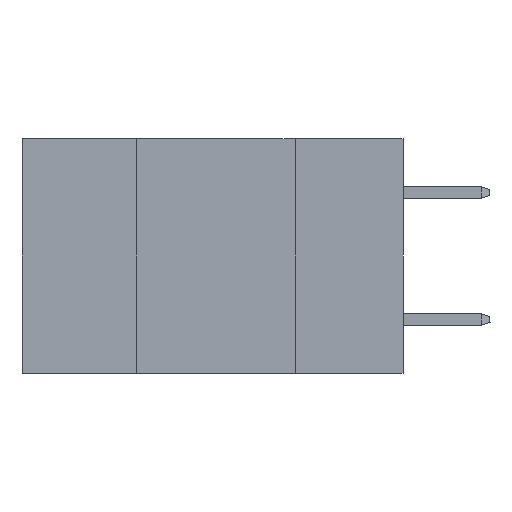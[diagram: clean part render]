
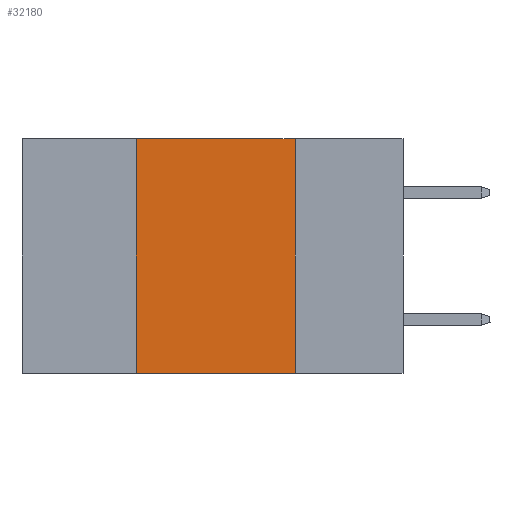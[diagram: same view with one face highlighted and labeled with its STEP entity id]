
A CAD part, left-side view. The second image highlights one B-rep face of the part: STEP entity #32180.
In plain terms, the highlighted planar face has unit normal (-1, 0, 0).
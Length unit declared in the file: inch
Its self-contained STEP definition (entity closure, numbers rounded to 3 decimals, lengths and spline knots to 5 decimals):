
#2008 = VERTEX_POINT ( 'NONE', #32092 ) ;
#3307 = CARTESIAN_POINT ( 'NONE',  ( 0., 0.17, 0. ) ) ;
#3973 = ORIENTED_EDGE ( 'NONE', *, *, #20197, .F. ) ;
#4289 = VERTEX_POINT ( 'NONE', #24339 ) ;
#4741 = LINE ( 'NONE', #33515, #11159 ) ;
#5116 = DIRECTION ( 'NONE',  ( 1., 0., 0. ) ) ;
#5204 = VECTOR ( 'NONE', #11372, 39.37008 ) ;
#5494 = DIRECTION ( 'NONE',  ( 0., -1., 0. ) ) ;
#6930 = CARTESIAN_POINT ( 'NONE',  ( 0., 0.6, -0.37 ) ) ;
#7945 = EDGE_CURVE ( 'NONE', #23927, #22514, #4741, .T. ) ;
#10489 = ORIENTED_EDGE ( 'NONE', *, *, #19503, .F. ) ;
#11159 = VECTOR ( 'NONE', #19785, 39.37008 ) ;
#11293 = VECTOR ( 'NONE', #5494, 39.37008 ) ;
#11372 = DIRECTION ( 'NONE',  ( 0., 0., -1. ) ) ;
#11696 = LINE ( 'NONE', #3307, #5204 ) ;
#14793 = LINE ( 'NONE', #6930, #11293 ) ;
#15014 = ORIENTED_EDGE ( 'NONE', *, *, #7945, .F. ) ;
#15033 = DIRECTION ( 'NONE',  ( 0., 0., -1. ) ) ;
#15169 = DIRECTION ( 'NONE',  ( 0., -1., 0. ) ) ;
#17349 = AXIS2_PLACEMENT_3D ( 'NONE', #28578, #5116, #15033 ) ;
#17660 = ORIENTED_EDGE ( 'NONE', *, *, #23368, .T. ) ;
#18107 = PLANE ( 'NONE',  #17349 ) ;
#19369 = VECTOR ( 'NONE', #15169, 39.37008 ) ;
#19503 = EDGE_CURVE ( 'NONE', #22514, #2008, #22879, .T. ) ;
#19785 = DIRECTION ( 'NONE',  ( 0., 0., 1. ) ) ;
#20197 = EDGE_CURVE ( 'NONE', #2008, #4289, #11696, .T. ) ;
#22514 = VERTEX_POINT ( 'NONE', #22914 ) ;
#22879 = LINE ( 'NONE', #33334, #19369 ) ;
#22914 = CARTESIAN_POINT ( 'NONE',  ( 0., 0.42, 0. ) ) ;
#23368 = EDGE_CURVE ( 'NONE', #23927, #4289, #14793, .T. ) ;
#23927 = VERTEX_POINT ( 'NONE', #29607 ) ;
#24339 = CARTESIAN_POINT ( 'NONE',  ( 0., 0.17, -0.37 ) ) ;
#28412 = FACE_OUTER_BOUND ( 'NONE', #33685, .T. ) ;
#28578 = CARTESIAN_POINT ( 'NONE',  ( 0., 0.6, 0. ) ) ;
#29607 = CARTESIAN_POINT ( 'NONE',  ( 0., 0.42, -0.37 ) ) ;
#32092 = CARTESIAN_POINT ( 'NONE',  ( 0., 0.17, 0. ) ) ;
#32180 = ADVANCED_FACE ( 'NONE', ( #28412 ), #18107, .F. ) ;
#33334 = CARTESIAN_POINT ( 'NONE',  ( 0., 0.6, 0. ) ) ;
#33515 = CARTESIAN_POINT ( 'NONE',  ( 0., 0.42, 0. ) ) ;
#33685 = EDGE_LOOP ( 'NONE', ( #3973, #10489, #15014, #17660 ) ) ;
